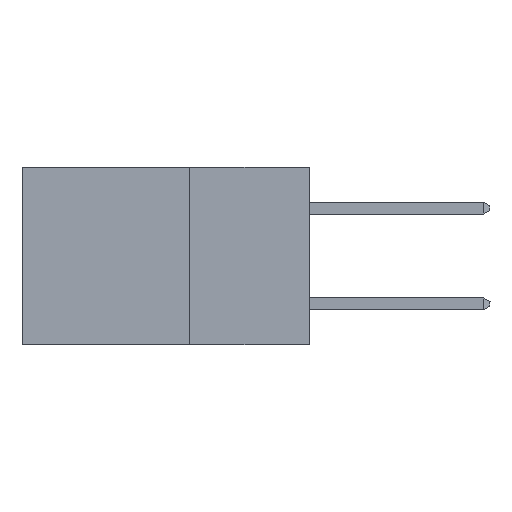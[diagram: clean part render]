
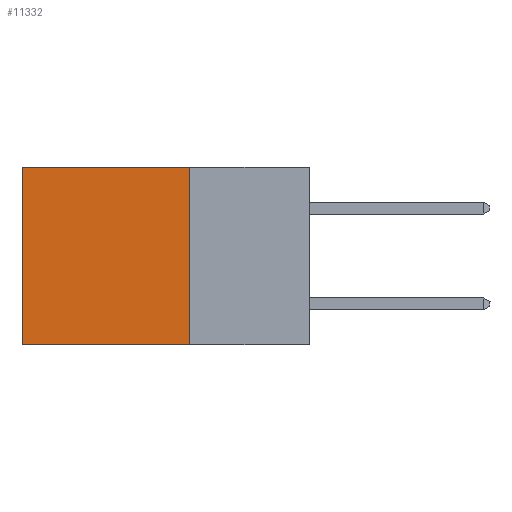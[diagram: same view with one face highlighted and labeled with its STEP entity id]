
A CAD part, left-side view. The second image highlights one B-rep face of the part: STEP entity #11332.
In plain terms, the highlighted planar face has unit normal (-1, 0, 0).
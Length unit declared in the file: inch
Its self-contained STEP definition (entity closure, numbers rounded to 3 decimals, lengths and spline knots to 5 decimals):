
#406 = DIRECTION ( 'NONE',  ( 0., 1., 0. ) ) ;
#1898 = VECTOR ( 'NONE', #14121, 39.37008 ) ;
#1979 = PLANE ( 'NONE',  #38771 ) ;
#2263 = EDGE_LOOP ( 'NONE', ( #28203, #38896, #12530, #15811 ) ) ;
#6685 = CARTESIAN_POINT ( 'NONE',  ( 0.2875, 0.25, 0. ) ) ;
#7193 = CARTESIAN_POINT ( 'NONE',  ( 0.2875, 0.25, 0. ) ) ;
#7943 = CARTESIAN_POINT ( 'NONE',  ( 0.2875, 0.6, -0.37 ) ) ;
#8263 = CARTESIAN_POINT ( 'NONE',  ( 0.2875, 0.25, 0. ) ) ;
#11264 = VERTEX_POINT ( 'NONE', #8263 ) ;
#11332 = ADVANCED_FACE ( 'NONE', ( #19817 ), #1979, .F. ) ;
#12530 = ORIENTED_EDGE ( 'NONE', *, *, #18906, .F. ) ;
#13510 = CARTESIAN_POINT ( 'NONE',  ( 0.2875, 0.25, -0.37 ) ) ;
#14121 = DIRECTION ( 'NONE',  ( 0., 0., -1. ) ) ;
#15388 = EDGE_CURVE ( 'NONE', #15667, #24907, #22785, .T. ) ;
#15667 = VERTEX_POINT ( 'NONE', #13510 ) ;
#15811 = ORIENTED_EDGE ( 'NONE', *, *, #45362, .T. ) ;
#16136 = CARTESIAN_POINT ( 'NONE',  ( 0.2875, 0.25, 0. ) ) ;
#17305 = VERTEX_POINT ( 'NONE', #20181 ) ;
#18906 = EDGE_CURVE ( 'NONE', #11264, #15667, #38918, .T. ) ;
#19817 = FACE_OUTER_BOUND ( 'NONE', #2263, .T. ) ;
#20181 = CARTESIAN_POINT ( 'NONE',  ( 0.2875, 0.6, 0. ) ) ;
#22785 = LINE ( 'NONE', #40160, #40431 ) ;
#24907 = VERTEX_POINT ( 'NONE', #7943 ) ;
#26587 = VECTOR ( 'NONE', #42631, 39.37008 ) ;
#26781 = DIRECTION ( 'NONE',  ( 0., 0., -1. ) ) ;
#28203 = ORIENTED_EDGE ( 'NONE', *, *, #33629, .T. ) ;
#31242 = LINE ( 'NONE', #6685, #41443 ) ;
#31720 = LINE ( 'NONE', #35187, #1898 ) ;
#33629 = EDGE_CURVE ( 'NONE', #17305, #24907, #31720, .T. ) ;
#35187 = CARTESIAN_POINT ( 'NONE',  ( 0.2875, 0.6, 0. ) ) ;
#38771 = AXIS2_PLACEMENT_3D ( 'NONE', #16136, #44388, #26781 ) ;
#38896 = ORIENTED_EDGE ( 'NONE', *, *, #15388, .F. ) ;
#38918 = LINE ( 'NONE', #7193, #26587 ) ;
#40160 = CARTESIAN_POINT ( 'NONE',  ( 0.2875, 0.25, -0.37 ) ) ;
#40431 = VECTOR ( 'NONE', #43648, 39.37008 ) ;
#41443 = VECTOR ( 'NONE', #406, 39.37008 ) ;
#42631 = DIRECTION ( 'NONE',  ( 0., 0., -1. ) ) ;
#43648 = DIRECTION ( 'NONE',  ( 0., 1., 0. ) ) ;
#44388 = DIRECTION ( 'NONE',  ( 1., 0., 0. ) ) ;
#45362 = EDGE_CURVE ( 'NONE', #11264, #17305, #31242, .T. ) ;
